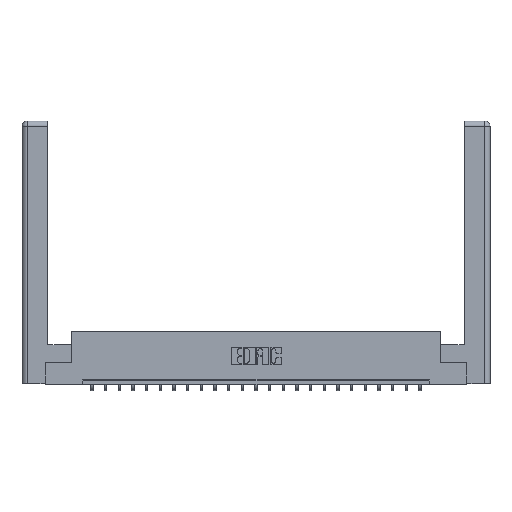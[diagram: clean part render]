
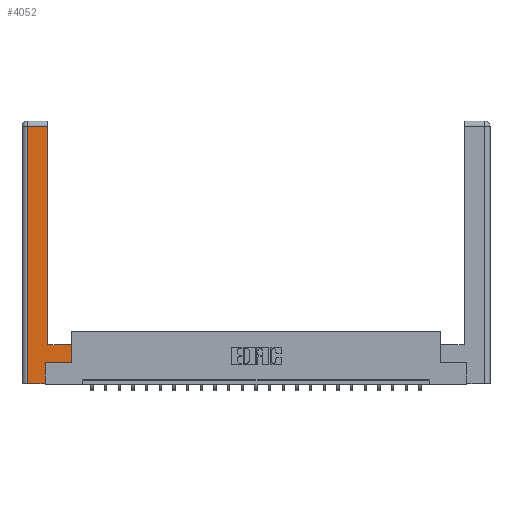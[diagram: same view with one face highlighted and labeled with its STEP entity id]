
A CAD part, top view. The second image highlights one B-rep face of the part: STEP entity #4052.
In plain terms, the highlighted planar face has unit normal (0, 0, 1).
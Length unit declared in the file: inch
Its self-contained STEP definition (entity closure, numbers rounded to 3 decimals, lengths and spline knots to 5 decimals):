
#721 = CARTESIAN_POINT ( 'NONE',  ( 0.565, 0.45, 0. ) ) ;
#1033 = CARTESIAN_POINT ( 'NONE',  ( 0.265, 0.245, 0. ) ) ;
#1043 = EDGE_CURVE ( 'NONE', #22184, #17954, #15297, .T. ) ;
#1147 = ORIENTED_EDGE ( 'NONE', *, *, #1299, .T. ) ;
#1299 = EDGE_CURVE ( 'NONE', #15489, #22184, #15849, .T. ) ;
#1451 = LINE ( 'NONE', #1961, #6273 ) ;
#1797 = VECTOR ( 'NONE', #11589, 39.37008 ) ;
#1961 = CARTESIAN_POINT ( 'NONE',  ( 0.295, 0.45, 0. ) ) ;
#2561 = EDGE_CURVE ( 'NONE', #5587, #6714, #14868, .T. ) ;
#2826 = EDGE_CURVE ( 'NONE', #17954, #5587, #5764, .T. ) ;
#2866 = DIRECTION ( 'NONE',  ( 0., 1., 0. ) ) ;
#3259 = ORIENTED_EDGE ( 'NONE', *, *, #18870, .T. ) ;
#4039 = CARTESIAN_POINT ( 'NONE',  ( 0.265, 0., 0. ) ) ;
#4052 = ADVANCED_FACE ( 'NONE', ( #23031 ), #6028, .F. ) ;
#4332 = LINE ( 'NONE', #19248, #9394 ) ;
#5115 = CARTESIAN_POINT ( 'NONE',  ( 0.0615, 0., 0. ) ) ;
#5255 = CARTESIAN_POINT ( 'NONE',  ( 0.265, 0.245, 0. ) ) ;
#5442 = DIRECTION ( 'NONE',  ( -1., 0., 0. ) ) ;
#5587 = VERTEX_POINT ( 'NONE', #19693 ) ;
#5764 = LINE ( 'NONE', #15682, #19134 ) ;
#5870 = ORIENTED_EDGE ( 'NONE', *, *, #12971, .T. ) ;
#6028 = PLANE ( 'NONE',  #6375 ) ;
#6270 = DIRECTION ( 'NONE',  ( 0., 0., -1. ) ) ;
#6273 = VECTOR ( 'NONE', #5442, 39.37008 ) ;
#6375 = AXIS2_PLACEMENT_3D ( 'NONE', #20560, #6270, #9666 ) ;
#6714 = VERTEX_POINT ( 'NONE', #721 ) ;
#6785 = CARTESIAN_POINT ( 'NONE',  ( 0.0615, 2.94, 0. ) ) ;
#7477 = CARTESIAN_POINT ( 'NONE',  ( 0.265, 0., 0. ) ) ;
#8852 = ORIENTED_EDGE ( 'NONE', *, *, #2826, .T. ) ;
#9394 = VECTOR ( 'NONE', #13601, 39.37008 ) ;
#9477 = DIRECTION ( 'NONE',  ( 0., 1., 0. ) ) ;
#9666 = DIRECTION ( 'NONE',  ( -1., 0., 0. ) ) ;
#10000 = ORIENTED_EDGE ( 'NONE', *, *, #19399, .T. ) ;
#10221 = DIRECTION ( 'NONE',  ( -1., 0., 0. ) ) ;
#11232 = ORIENTED_EDGE ( 'NONE', *, *, #1043, .T. ) ;
#11414 = DIRECTION ( 'NONE',  ( 1., 0., 0. ) ) ;
#11589 = DIRECTION ( 'NONE',  ( 0., -1., 0. ) ) ;
#12714 = CARTESIAN_POINT ( 'NONE',  ( 0.295, 0.45, 0. ) ) ;
#12769 = EDGE_LOOP ( 'NONE', ( #3259, #5870, #10000, #1147, #11232, #8852, #16635, #23084 ) ) ;
#12971 = EDGE_CURVE ( 'NONE', #16031, #17185, #23473, .T. ) ;
#13601 = DIRECTION ( 'NONE',  ( 0., 1., 0. ) ) ;
#14002 = VECTOR ( 'NONE', #9477, 39.37008 ) ;
#14868 = LINE ( 'NONE', #14897, #14002 ) ;
#14897 = CARTESIAN_POINT ( 'NONE',  ( 0.565, 0.45, 0. ) ) ;
#15297 = LINE ( 'NONE', #1033, #15564 ) ;
#15489 = VERTEX_POINT ( 'NONE', #5115 ) ;
#15564 = VECTOR ( 'NONE', #2866, 39.37008 ) ;
#15682 = CARTESIAN_POINT ( 'NONE',  ( 0.565, 0.245, 0. ) ) ;
#15849 = LINE ( 'NONE', #4039, #23501 ) ;
#16031 = VERTEX_POINT ( 'NONE', #22945 ) ;
#16635 = ORIENTED_EDGE ( 'NONE', *, *, #2561, .T. ) ;
#16867 = EDGE_CURVE ( 'NONE', #6714, #19108, #1451, .T. ) ;
#17185 = VERTEX_POINT ( 'NONE', #6785 ) ;
#17698 = DIRECTION ( 'NONE',  ( 1., 0., 0. ) ) ;
#17954 = VERTEX_POINT ( 'NONE', #5255 ) ;
#18870 = EDGE_CURVE ( 'NONE', #19108, #16031, #4332, .T. ) ;
#19108 = VERTEX_POINT ( 'NONE', #12714 ) ;
#19134 = VECTOR ( 'NONE', #17698, 39.37008 ) ;
#19248 = CARTESIAN_POINT ( 'NONE',  ( 0.295, 3., 0. ) ) ;
#19399 = EDGE_CURVE ( 'NONE', #17185, #15489, #20524, .T. ) ;
#19693 = CARTESIAN_POINT ( 'NONE',  ( 0.565, 0.245, 0. ) ) ;
#20524 = LINE ( 'NONE', #22626, #1797 ) ;
#20560 = CARTESIAN_POINT ( 'NONE',  ( 0., 0., 0. ) ) ;
#21105 = CARTESIAN_POINT ( 'NONE',  ( 0.0615, 2.94, 0. ) ) ;
#21206 = VECTOR ( 'NONE', #10221, 39.37008 ) ;
#22184 = VERTEX_POINT ( 'NONE', #7477 ) ;
#22626 = CARTESIAN_POINT ( 'NONE',  ( 0.0615, 0., 0. ) ) ;
#22945 = CARTESIAN_POINT ( 'NONE',  ( 0.295, 2.94, 0. ) ) ;
#23031 = FACE_OUTER_BOUND ( 'NONE', #12769, .T. ) ;
#23084 = ORIENTED_EDGE ( 'NONE', *, *, #16867, .T. ) ;
#23473 = LINE ( 'NONE', #21105, #21206 ) ;
#23501 = VECTOR ( 'NONE', #11414, 39.37008 ) ;
